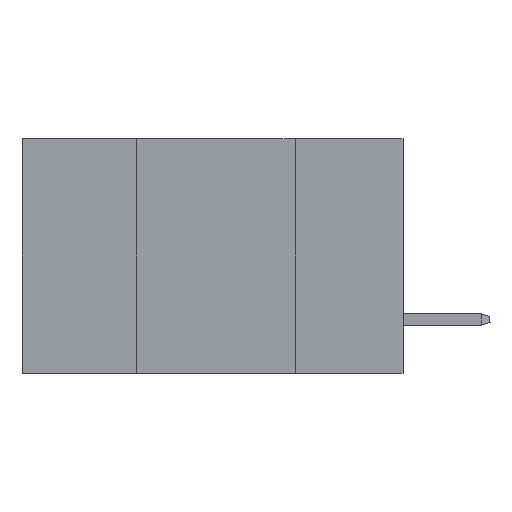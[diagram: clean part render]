
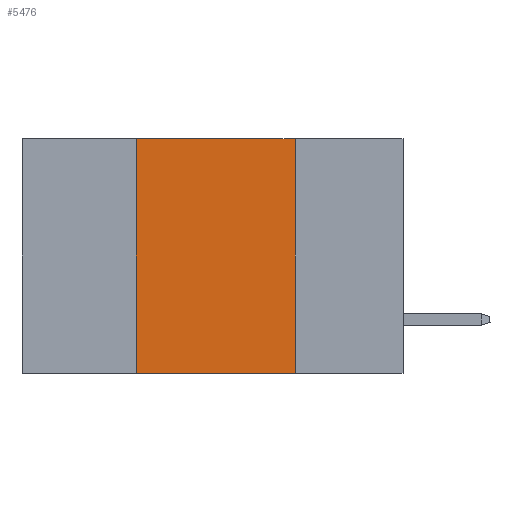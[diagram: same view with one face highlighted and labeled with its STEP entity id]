
A CAD part, left-side view. The second image highlights one B-rep face of the part: STEP entity #5476.
In plain terms, the highlighted planar face has unit normal (-1, 0, 0).
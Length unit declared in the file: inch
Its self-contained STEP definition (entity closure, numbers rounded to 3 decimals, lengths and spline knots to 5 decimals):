
#72 = VECTOR ( 'NONE', #16478, 39.37008 ) ;
#83 = EDGE_LOOP ( 'NONE', ( #2390, #15957, #20165, #9314 ) ) ;
#107 = EDGE_CURVE ( 'NONE', #4443, #9582, #21350, .T. ) ;
#240 = VERTEX_POINT ( 'NONE', #21898 ) ;
#303 = CARTESIAN_POINT ( 'NONE',  ( 0., 0.6, -0.37 ) ) ;
#1586 = CARTESIAN_POINT ( 'NONE',  ( 0., 0.17, 0. ) ) ;
#2390 = ORIENTED_EDGE ( 'NONE', *, *, #11671, .F. ) ;
#2988 = CARTESIAN_POINT ( 'NONE',  ( 0., 0.17, 0. ) ) ;
#4443 = VERTEX_POINT ( 'NONE', #7702 ) ;
#4792 = DIRECTION ( 'NONE',  ( 0., 0., 1. ) ) ;
#5476 = ADVANCED_FACE ( 'NONE', ( #20941 ), #7103, .F. ) ;
#6194 = CARTESIAN_POINT ( 'NONE',  ( 0., 0.6, 0. ) ) ;
#7103 = PLANE ( 'NONE',  #15416 ) ;
#7547 = CARTESIAN_POINT ( 'NONE',  ( 0., 0.6, 0. ) ) ;
#7702 = CARTESIAN_POINT ( 'NONE',  ( 0., 0.42, 0. ) ) ;
#8246 = VECTOR ( 'NONE', #4792, 39.37008 ) ;
#8718 = LINE ( 'NONE', #303, #16432 ) ;
#8870 = DIRECTION ( 'NONE',  ( 0., 0., -1. ) ) ;
#9314 = ORIENTED_EDGE ( 'NONE', *, *, #20388, .T. ) ;
#9582 = VERTEX_POINT ( 'NONE', #1586 ) ;
#9646 = LINE ( 'NONE', #14516, #8246 ) ;
#9841 = LINE ( 'NONE', #2988, #72 ) ;
#10952 = VERTEX_POINT ( 'NONE', #21890 ) ;
#11671 = EDGE_CURVE ( 'NONE', #9582, #10952, #9841, .T. ) ;
#12919 = DIRECTION ( 'NONE',  ( 0., -1., 0. ) ) ;
#14516 = CARTESIAN_POINT ( 'NONE',  ( 0., 0.42, 0. ) ) ;
#15045 = VECTOR ( 'NONE', #12919, 39.37008 ) ;
#15416 = AXIS2_PLACEMENT_3D ( 'NONE', #7547, #21056, #8870 ) ;
#15957 = ORIENTED_EDGE ( 'NONE', *, *, #107, .F. ) ;
#16432 = VECTOR ( 'NONE', #18905, 39.37008 ) ;
#16478 = DIRECTION ( 'NONE',  ( 0., 0., -1. ) ) ;
#17823 = EDGE_CURVE ( 'NONE', #240, #4443, #9646, .T. ) ;
#18905 = DIRECTION ( 'NONE',  ( 0., -1., 0. ) ) ;
#20165 = ORIENTED_EDGE ( 'NONE', *, *, #17823, .F. ) ;
#20388 = EDGE_CURVE ( 'NONE', #240, #10952, #8718, .T. ) ;
#20941 = FACE_OUTER_BOUND ( 'NONE', #83, .T. ) ;
#21056 = DIRECTION ( 'NONE',  ( 1., 0., 0. ) ) ;
#21350 = LINE ( 'NONE', #6194, #15045 ) ;
#21890 = CARTESIAN_POINT ( 'NONE',  ( 0., 0.17, -0.37 ) ) ;
#21898 = CARTESIAN_POINT ( 'NONE',  ( 0., 0.42, -0.37 ) ) ;
